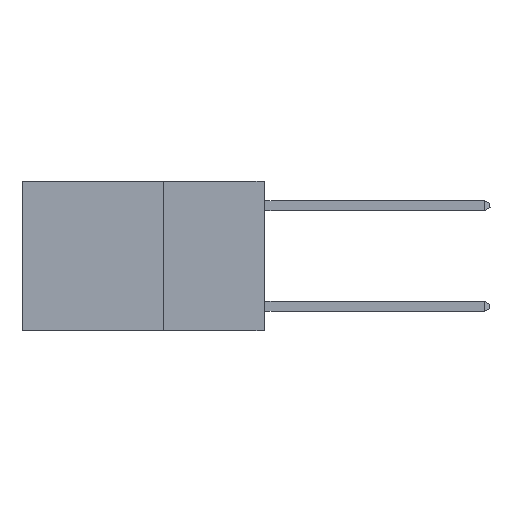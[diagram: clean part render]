
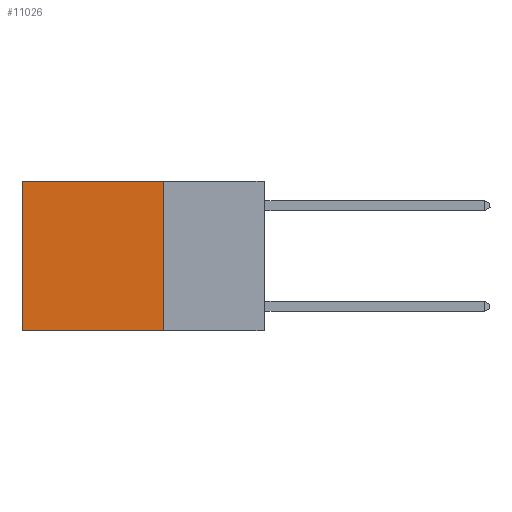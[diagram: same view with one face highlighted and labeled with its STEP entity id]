
A CAD part, left-side view. The second image highlights one B-rep face of the part: STEP entity #11026.
In plain terms, the highlighted planar face has unit normal (-1, 0, 0).
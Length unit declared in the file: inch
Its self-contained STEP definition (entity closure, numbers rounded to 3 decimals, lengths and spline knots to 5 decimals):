
#97 = VERTEX_POINT ( 'NONE', #3148 ) ;
#316 = DIRECTION ( 'NONE',  ( 0., 0., -1. ) ) ;
#424 = VERTEX_POINT ( 'NONE', #7054 ) ;
#1485 = CARTESIAN_POINT ( 'NONE',  ( 0.2625, 0.6, 0. ) ) ;
#2188 = ORIENTED_EDGE ( 'NONE', *, *, #11044, .T. ) ;
#2440 = CARTESIAN_POINT ( 'NONE',  ( 0.2625, 0.6, -0.37 ) ) ;
#3148 = CARTESIAN_POINT ( 'NONE',  ( 0.2625, 0.25, -0.37 ) ) ;
#3631 = LINE ( 'NONE', #14564, #3969 ) ;
#3947 = EDGE_CURVE ( 'NONE', #97, #9580, #3631, .T. ) ;
#3969 = VECTOR ( 'NONE', #5961, 39.37008 ) ;
#4495 = ORIENTED_EDGE ( 'NONE', *, *, #9831, .F. ) ;
#5724 = ORIENTED_EDGE ( 'NONE', *, *, #11284, .T. ) ;
#5892 = EDGE_LOOP ( 'NONE', ( #2188, #13950, #4495, #5724 ) ) ;
#5943 = VECTOR ( 'NONE', #316, 39.37008 ) ;
#5961 = DIRECTION ( 'NONE',  ( 0., 1., 0. ) ) ;
#6868 = LINE ( 'NONE', #1485, #5943 ) ;
#6914 = VECTOR ( 'NONE', #7838, 39.37008 ) ;
#7054 = CARTESIAN_POINT ( 'NONE',  ( 0.2625, 0.25, 0. ) ) ;
#7481 = VERTEX_POINT ( 'NONE', #9759 ) ;
#7594 = PLANE ( 'NONE',  #10853 ) ;
#7624 = VECTOR ( 'NONE', #8232, 39.37008 ) ;
#7838 = DIRECTION ( 'NONE',  ( 0., 0., -1. ) ) ;
#7906 = DIRECTION ( 'NONE',  ( 1., 0., 0. ) ) ;
#8232 = DIRECTION ( 'NONE',  ( 0., 1., 0. ) ) ;
#8252 = LINE ( 'NONE', #9604, #6914 ) ;
#9149 = DIRECTION ( 'NONE',  ( 0., 0., -1. ) ) ;
#9580 = VERTEX_POINT ( 'NONE', #2440 ) ;
#9604 = CARTESIAN_POINT ( 'NONE',  ( 0.2625, 0.25, 0. ) ) ;
#9759 = CARTESIAN_POINT ( 'NONE',  ( 0.2625, 0.6, 0. ) ) ;
#9831 = EDGE_CURVE ( 'NONE', #424, #97, #8252, .T. ) ;
#10853 = AXIS2_PLACEMENT_3D ( 'NONE', #14200, #7906, #9149 ) ;
#11026 = ADVANCED_FACE ( 'NONE', ( #12044 ), #7594, .F. ) ;
#11044 = EDGE_CURVE ( 'NONE', #7481, #9580, #6868, .T. ) ;
#11284 = EDGE_CURVE ( 'NONE', #424, #7481, #13567, .T. ) ;
#11359 = CARTESIAN_POINT ( 'NONE',  ( 0.2625, 0.25, 0. ) ) ;
#12044 = FACE_OUTER_BOUND ( 'NONE', #5892, .T. ) ;
#13567 = LINE ( 'NONE', #11359, #7624 ) ;
#13950 = ORIENTED_EDGE ( 'NONE', *, *, #3947, .F. ) ;
#14200 = CARTESIAN_POINT ( 'NONE',  ( 0.2625, 0.25, 0. ) ) ;
#14564 = CARTESIAN_POINT ( 'NONE',  ( 0.2625, 0.25, -0.37 ) ) ;
